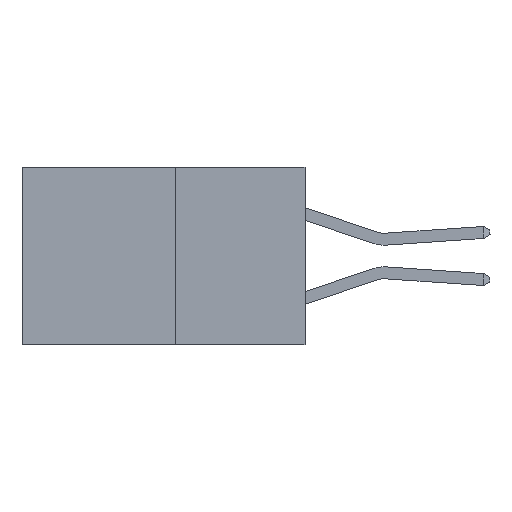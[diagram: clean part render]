
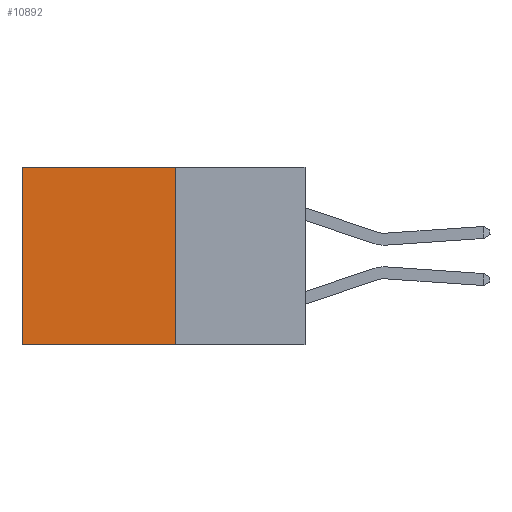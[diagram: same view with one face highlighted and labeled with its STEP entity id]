
A CAD part, left-side view. The second image highlights one B-rep face of the part: STEP entity #10892.
In plain terms, the highlighted planar face has unit normal (-1, 0, 0).
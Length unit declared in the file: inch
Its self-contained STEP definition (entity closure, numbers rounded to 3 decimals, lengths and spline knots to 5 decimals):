
#208 = CARTESIAN_POINT ( 'NONE',  ( 0.277, 0.27, 0. ) ) ;
#361 = CARTESIAN_POINT ( 'NONE',  ( 0.277, 0.59, -0.37 ) ) ;
#530 = VERTEX_POINT ( 'NONE', #11125 ) ;
#817 = LINE ( 'NONE', #7291, #8529 ) ;
#950 = VECTOR ( 'NONE', #9532, 39.37008 ) ;
#1463 = EDGE_CURVE ( 'NONE', #9827, #9190, #817, .T. ) ;
#1483 = ORIENTED_EDGE ( 'NONE', *, *, #5304, .T. ) ;
#1631 = DIRECTION ( 'NONE',  ( 0., 1., 0. ) ) ;
#1706 = ORIENTED_EDGE ( 'NONE', *, *, #12590, .T. ) ;
#2529 = VECTOR ( 'NONE', #7211, 39.37008 ) ;
#2957 = PLANE ( 'NONE',  #8079 ) ;
#3022 = CARTESIAN_POINT ( 'NONE',  ( 0.277, 0.59, 0. ) ) ;
#3330 = FACE_OUTER_BOUND ( 'NONE', #8101, .T. ) ;
#3588 = LINE ( 'NONE', #9516, #950 ) ;
#3921 = DIRECTION ( 'NONE',  ( 1., 0., 0. ) ) ;
#3942 = EDGE_CURVE ( 'NONE', #530, #9827, #3588, .T. ) ;
#4508 = LINE ( 'NONE', #208, #2529 ) ;
#5304 = EDGE_CURVE ( 'NONE', #8389, #9190, #12340, .T. ) ;
#5874 = ORIENTED_EDGE ( 'NONE', *, *, #1463, .F. ) ;
#6314 = CARTESIAN_POINT ( 'NONE',  ( 0.277, 0.27, -0.37 ) ) ;
#7211 = DIRECTION ( 'NONE',  ( 0., 1., 0. ) ) ;
#7291 = CARTESIAN_POINT ( 'NONE',  ( 0.277, 0.27, -0.37 ) ) ;
#7494 = VECTOR ( 'NONE', #10784, 39.37008 ) ;
#8079 = AXIS2_PLACEMENT_3D ( 'NONE', #9991, #3921, #10962 ) ;
#8101 = EDGE_LOOP ( 'NONE', ( #1483, #5874, #8766, #1706 ) ) ;
#8389 = VERTEX_POINT ( 'NONE', #3022 ) ;
#8422 = CARTESIAN_POINT ( 'NONE',  ( 0.277, 0.59, -0.37 ) ) ;
#8529 = VECTOR ( 'NONE', #1631, 39.37008 ) ;
#8766 = ORIENTED_EDGE ( 'NONE', *, *, #3942, .F. ) ;
#9190 = VERTEX_POINT ( 'NONE', #8422 ) ;
#9516 = CARTESIAN_POINT ( 'NONE',  ( 0.277, 0.27, -0.37 ) ) ;
#9532 = DIRECTION ( 'NONE',  ( 0., 0., -1. ) ) ;
#9827 = VERTEX_POINT ( 'NONE', #6314 ) ;
#9991 = CARTESIAN_POINT ( 'NONE',  ( 0.277, 0.27, -0.37 ) ) ;
#10784 = DIRECTION ( 'NONE',  ( 0., 0., -1. ) ) ;
#10892 = ADVANCED_FACE ( 'NONE', ( #3330 ), #2957, .F. ) ;
#10962 = DIRECTION ( 'NONE',  ( 0., 0., -1. ) ) ;
#11125 = CARTESIAN_POINT ( 'NONE',  ( 0.277, 0.27, 0. ) ) ;
#12340 = LINE ( 'NONE', #361, #7494 ) ;
#12590 = EDGE_CURVE ( 'NONE', #530, #8389, #4508, .T. ) ;
